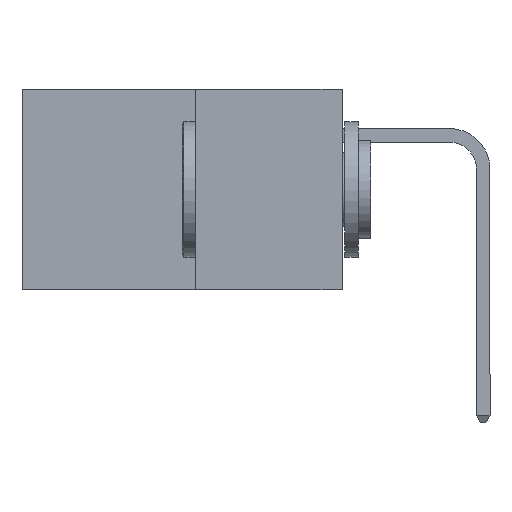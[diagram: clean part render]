
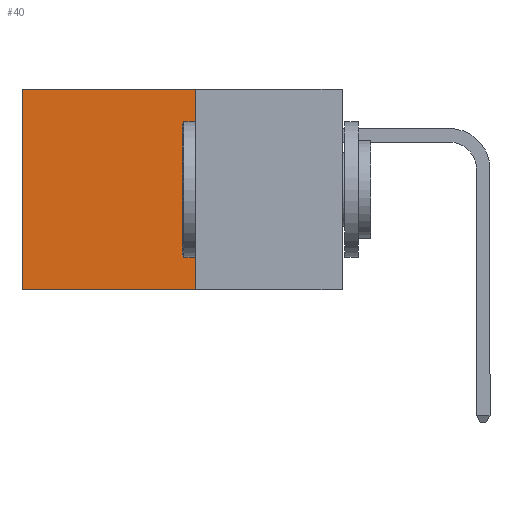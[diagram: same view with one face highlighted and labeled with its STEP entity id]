
A CAD part, left-side view. The second image highlights one B-rep face of the part: STEP entity #40.
In plain terms, the highlighted planar face has unit normal (-1, 0, 0).
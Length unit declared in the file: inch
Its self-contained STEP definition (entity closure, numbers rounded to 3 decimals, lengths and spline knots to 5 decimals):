
#40 = ADVANCED_FACE ( 'NONE', ( #2487 ), #1843, .F. ) ;
#429 = CARTESIAN_POINT ( 'NONE',  ( 0.277, 0.27, 0. ) ) ;
#582 = CARTESIAN_POINT ( 'NONE',  ( 0.277, 0.59, -0.37 ) ) ;
#843 = LINE ( 'NONE', #429, #7773 ) ;
#1111 = VECTOR ( 'NONE', #4631, 39.37008 ) ;
#1116 = VECTOR ( 'NONE', #8287, 39.37008 ) ;
#1171 = CARTESIAN_POINT ( 'NONE',  ( 0.277, 0.27, -0.37 ) ) ;
#1283 = CARTESIAN_POINT ( 'NONE',  ( 0.277, 0.59, 0. ) ) ;
#1610 = ORIENTED_EDGE ( 'NONE', *, *, #3933, .T. ) ;
#1843 = PLANE ( 'NONE',  #5785 ) ;
#2053 = EDGE_CURVE ( 'NONE', #5722, #5201, #2252, .T. ) ;
#2183 = EDGE_LOOP ( 'NONE', ( #1610, #5109, #7032, #4378 ) ) ;
#2252 = LINE ( 'NONE', #6910, #5555 ) ;
#2487 = FACE_OUTER_BOUND ( 'NONE', #2183, .T. ) ;
#2819 = VERTEX_POINT ( 'NONE', #1283 ) ;
#3494 = EDGE_CURVE ( 'NONE', #5201, #5342, #6362, .T. ) ;
#3817 = CARTESIAN_POINT ( 'NONE',  ( 0.277, 0.27, -0.37 ) ) ;
#3933 = EDGE_CURVE ( 'NONE', #2819, #5342, #4397, .T. ) ;
#4378 = ORIENTED_EDGE ( 'NONE', *, *, #8299, .T. ) ;
#4388 = DIRECTION ( 'NONE',  ( 0., 1., 0. ) ) ;
#4397 = LINE ( 'NONE', #582, #1111 ) ;
#4631 = DIRECTION ( 'NONE',  ( 0., 0., -1. ) ) ;
#5109 = ORIENTED_EDGE ( 'NONE', *, *, #3494, .F. ) ;
#5201 = VERTEX_POINT ( 'NONE', #3817 ) ;
#5342 = VERTEX_POINT ( 'NONE', #8250 ) ;
#5555 = VECTOR ( 'NONE', #6571, 39.37008 ) ;
#5722 = VERTEX_POINT ( 'NONE', #6794 ) ;
#5785 = AXIS2_PLACEMENT_3D ( 'NONE', #8262, #6099, #7949 ) ;
#6099 = DIRECTION ( 'NONE',  ( 1., 0., 0. ) ) ;
#6362 = LINE ( 'NONE', #1171, #1116 ) ;
#6571 = DIRECTION ( 'NONE',  ( 0., 0., -1. ) ) ;
#6794 = CARTESIAN_POINT ( 'NONE',  ( 0.277, 0.27, 0. ) ) ;
#6910 = CARTESIAN_POINT ( 'NONE',  ( 0.277, 0.27, -0.37 ) ) ;
#7032 = ORIENTED_EDGE ( 'NONE', *, *, #2053, .F. ) ;
#7773 = VECTOR ( 'NONE', #4388, 39.37008 ) ;
#7949 = DIRECTION ( 'NONE',  ( 0., 0., -1. ) ) ;
#8250 = CARTESIAN_POINT ( 'NONE',  ( 0.277, 0.59, -0.37 ) ) ;
#8262 = CARTESIAN_POINT ( 'NONE',  ( 0.277, 0.27, -0.37 ) ) ;
#8287 = DIRECTION ( 'NONE',  ( 0., 1., 0. ) ) ;
#8299 = EDGE_CURVE ( 'NONE', #5722, #2819, #843, .T. ) ;
